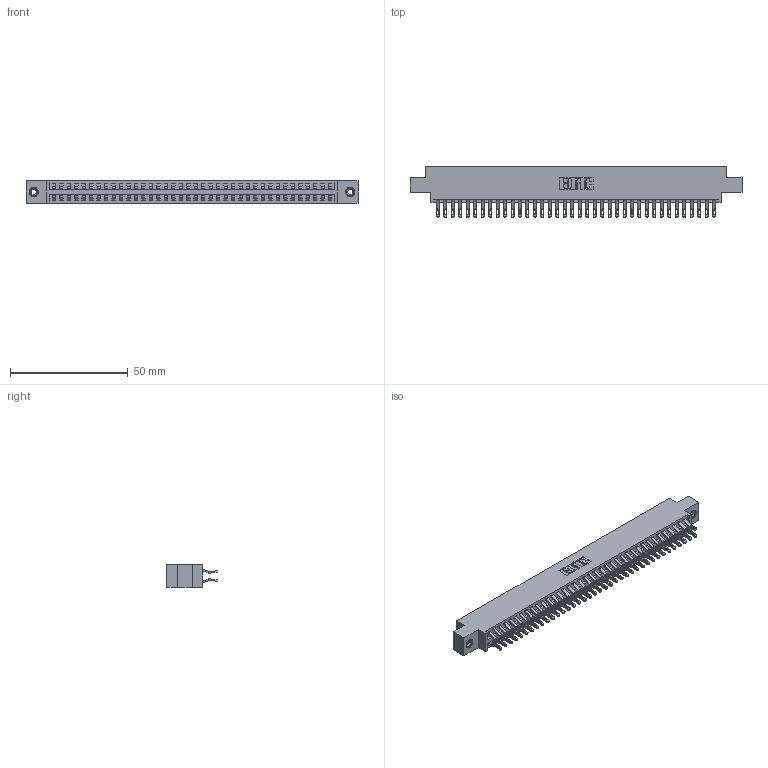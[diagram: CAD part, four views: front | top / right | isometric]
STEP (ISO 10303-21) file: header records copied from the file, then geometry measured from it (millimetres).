
FILE_DESCRIPTION (( 'STEP AP203' ), '1' );
FILE_NAME ('396-076-555-808.STEP', '2019-11-02T13:04:41', ( '' ), ( '' ), 'SwSTEP 2.0', 'SolidWorks 2016', '' );
FILE_SCHEMA (( 'CONFIG_CONTROL_DESIGN' ));
Length unit declared in the file: inch
Products named in the file (4): 346 Part_0.170 Offset - 0.156 Dia-TI; 345-292-001_555 Tail; 345-250-001_345-250-003-102; 396-076-555-808
Assembly tree (79 placements, depth 2):
  396-076-555-808
    346 Part_0.170 Offset - 0.156 Dia-TI
    345-292-001_555 Tail  x76
    345-250-001_345-250-003-102  x2
Bounding box: 141.22 x 21.46 x 9.4 mm (x, y, z)
Volume: 13799.3 mm3; surface area: 19890.7 mm2
Topology: 79 solids, 79 shells, 4594 faces, 14385 edges, 9582 vertices
Faces by surface type: plane 2620, cylinder 1958, cone 12, torus 4
Entity records: 26982 total; most frequent: CARTESIAN_POINT 4473, ORIENTED_EDGE 4370, DIRECTION 3987, EDGE_CURVE 2185, LINE 1861, VECTOR 1861, VERTEX_POINT 1452, AXIS2_PLACEMENT_3D 1063
